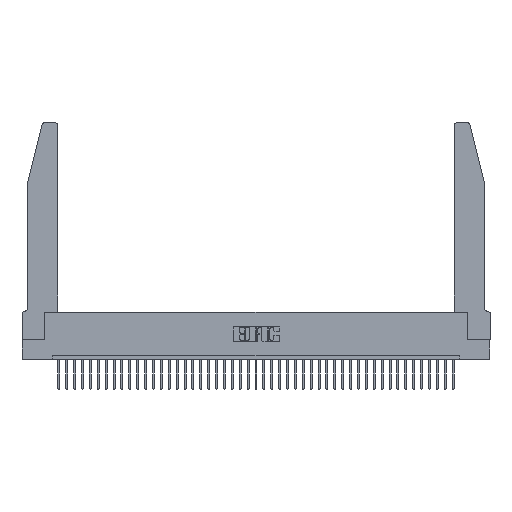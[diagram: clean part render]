
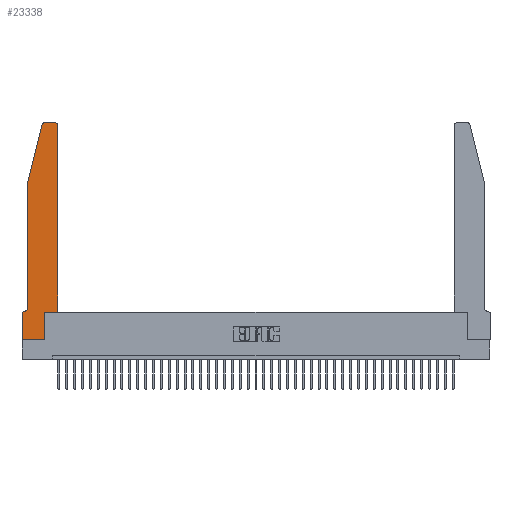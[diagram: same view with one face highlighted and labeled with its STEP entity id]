
A CAD part, top view. The second image highlights one B-rep face of the part: STEP entity #23338.
In plain terms, the highlighted planar face has unit normal (0, 0, 1).
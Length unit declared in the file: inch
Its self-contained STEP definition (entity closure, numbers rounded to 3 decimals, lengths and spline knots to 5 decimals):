
#655 = VERTEX_POINT ( 'NONE', #18500 ) ;
#844 = EDGE_CURVE ( 'NONE', #29490, #19747, #3680, .T. ) ;
#897 = DIRECTION ( 'NONE',  ( 0., -1., 0. ) ) ;
#1225 = VERTEX_POINT ( 'NONE', #5755 ) ;
#1467 = FACE_OUTER_BOUND ( 'NONE', #24844, .T. ) ;
#1492 = DIRECTION ( 'NONE',  ( 0., 0., 1. ) ) ;
#1796 = CARTESIAN_POINT ( 'NONE',  ( 0.284, 2.75, 0.37 ) ) ;
#1961 = CARTESIAN_POINT ( 'NONE',  ( 0.0755, 2., 0.37 ) ) ;
#2052 = VERTEX_POINT ( 'NONE', #10252 ) ;
#2252 = VECTOR ( 'NONE', #21838, 39.37008 ) ;
#2318 = CARTESIAN_POINT ( 'NONE',  ( 0.2605, 2.75, 0.37 ) ) ;
#2495 = VECTOR ( 'NONE', #20923, 39.37008 ) ;
#2794 = ORIENTED_EDGE ( 'NONE', *, *, #21121, .T. ) ;
#3680 = CIRCLE ( 'NONE', #6581, 0.03 ) ;
#4065 = CARTESIAN_POINT ( 'NONE',  ( 0., 0., 0.37 ) ) ;
#4233 = VECTOR ( 'NONE', #21711, 39.37008 ) ;
#5175 = CARTESIAN_POINT ( 'NONE',  ( 0.4505, 0.35, 0.37 ) ) ;
#5755 = CARTESIAN_POINT ( 'NONE',  ( 0.2865, 0.35, 0.37 ) ) ;
#6344 = LINE ( 'NONE', #2318, #2252 ) ;
#6581 = AXIS2_PLACEMENT_3D ( 'NONE', #23271, #13823, #37206 ) ;
#7173 = VERTEX_POINT ( 'NONE', #1796 ) ;
#7317 = LINE ( 'NONE', #12510, #4233 ) ;
#7359 = ORIENTED_EDGE ( 'NONE', *, *, #10147, .T. ) ;
#7855 = ORIENTED_EDGE ( 'NONE', *, *, #9364, .T. ) ;
#8074 = DIRECTION ( 'NONE',  ( 1., 0., 0. ) ) ;
#8273 = ORIENTED_EDGE ( 'NONE', *, *, #15355, .T. ) ;
#8410 = CARTESIAN_POINT ( 'NONE',  ( 0.4505, 0.35, 0.37 ) ) ;
#9364 = EDGE_CURVE ( 'NONE', #10448, #33351, #32750, .T. ) ;
#9763 = CARTESIAN_POINT ( 'NONE',  ( 0.284, 2.72, 0.37 ) ) ;
#10147 = EDGE_CURVE ( 'NONE', #38852, #29490, #27748, .T. ) ;
#10252 = CARTESIAN_POINT ( 'NONE',  ( 0.25487, 2.72718, 0.37 ) ) ;
#10448 = VERTEX_POINT ( 'NONE', #26435 ) ;
#11388 = VERTEX_POINT ( 'NONE', #17758 ) ;
#12142 = ORIENTED_EDGE ( 'NONE', *, *, #20381, .T. ) ;
#12510 = CARTESIAN_POINT ( 'NONE',  ( 0.0755, 2., 0.37 ) ) ;
#12698 = DIRECTION ( 'NONE',  ( 0., 1., 0. ) ) ;
#13823 = DIRECTION ( 'NONE',  ( 0., 0., 1. ) ) ;
#13905 = DIRECTION ( 'NONE',  ( 0., 0., 1. ) ) ;
#13908 = PLANE ( 'NONE',  #20901 ) ;
#14252 = LINE ( 'NONE', #28905, #28902 ) ;
#14485 = ORIENTED_EDGE ( 'NONE', *, *, #21116, .T. ) ;
#14889 = CARTESIAN_POINT ( 'NONE',  ( 0.4205, 2.75, 0.37 ) ) ;
#14927 = EDGE_CURVE ( 'NONE', #7173, #2052, #18191, .T. ) ;
#15355 = EDGE_CURVE ( 'NONE', #2052, #39242, #28479, .T. ) ;
#15704 = AXIS2_PLACEMENT_3D ( 'NONE', #33515, #37366, #37084 ) ;
#16388 = LINE ( 'NONE', #5175, #30599 ) ;
#17758 = CARTESIAN_POINT ( 'NONE',  ( 0.0755, 0.42, 0.37 ) ) ;
#18191 = CIRCLE ( 'NONE', #26035, 0.03 ) ;
#18500 = CARTESIAN_POINT ( 'NONE',  ( 0.0055, 0.35, 0.37 ) ) ;
#19199 = ORIENTED_EDGE ( 'NONE', *, *, #26691, .T. ) ;
#19747 = VERTEX_POINT ( 'NONE', #14889 ) ;
#20086 = DIRECTION ( 'NONE',  ( 1., 0., 0. ) ) ;
#20381 = EDGE_CURVE ( 'NONE', #11388, #655, #41296, .T. ) ;
#20901 = AXIS2_PLACEMENT_3D ( 'NONE', #23945, #1492, #8074 ) ;
#20923 = DIRECTION ( 'NONE',  ( 0., 1., 0. ) ) ;
#21116 = EDGE_CURVE ( 'NONE', #39242, #11388, #7317, .T. ) ;
#21121 = EDGE_CURVE ( 'NONE', #19747, #7173, #6344, .T. ) ;
#21711 = DIRECTION ( 'NONE',  ( 0., -1., 0. ) ) ;
#21838 = DIRECTION ( 'NONE',  ( -1., 0., 0. ) ) ;
#23271 = CARTESIAN_POINT ( 'NONE',  ( 0.4205, 2.72, 0.37 ) ) ;
#23338 = ADVANCED_FACE ( 'NONE', ( #1467 ), #13908, .T. ) ;
#23424 = CARTESIAN_POINT ( 'NONE',  ( 0., 0., 0.37 ) ) ;
#23945 = CARTESIAN_POINT ( 'NONE',  ( 0., 0.35, 0.37 ) ) ;
#24200 = VECTOR ( 'NONE', #897, 39.37008 ) ;
#24362 = DIRECTION ( 'NONE',  ( 1., 0., 0. ) ) ;
#24666 = ORIENTED_EDGE ( 'NONE', *, *, #38622, .T. ) ;
#24844 = EDGE_LOOP ( 'NONE', ( #2794, #31527, #8273, #14485, #12142, #19199, #7855, #34890, #40819, #24666, #7359, #34137 ) ) ;
#25403 = CARTESIAN_POINT ( 'NONE',  ( 0.0755, 0.35, 0.37 ) ) ;
#26035 = AXIS2_PLACEMENT_3D ( 'NONE', #9763, #13905, #20086 ) ;
#26435 = CARTESIAN_POINT ( 'NONE',  ( 0., 0.35, 0.37 ) ) ;
#26639 = EDGE_CURVE ( 'NONE', #29148, #1225, #14252, .T. ) ;
#26691 = EDGE_CURVE ( 'NONE', #655, #10448, #41616, .T. ) ;
#27676 = EDGE_CURVE ( 'NONE', #33351, #29148, #29787, .T. ) ;
#27748 = LINE ( 'NONE', #8410, #2495 ) ;
#28479 = LINE ( 'NONE', #1961, #36472 ) ;
#28902 = VECTOR ( 'NONE', #12698, 39.37008 ) ;
#28905 = CARTESIAN_POINT ( 'NONE',  ( 0.2865, 0.35, 0.37 ) ) ;
#29148 = VERTEX_POINT ( 'NONE', #35336 ) ;
#29490 = VERTEX_POINT ( 'NONE', #30052 ) ;
#29787 = LINE ( 'NONE', #38335, #36433 ) ;
#30015 = DIRECTION ( 'NONE',  ( -1., 0., 0. ) ) ;
#30052 = CARTESIAN_POINT ( 'NONE',  ( 0.4505, 2.72, 0.37 ) ) ;
#30215 = CARTESIAN_POINT ( 'NONE',  ( 0.4505, 0.35, 0.37 ) ) ;
#30599 = VECTOR ( 'NONE', #24362, 39.37008 ) ;
#31393 = DIRECTION ( 'NONE',  ( 1., 0., 0. ) ) ;
#31527 = ORIENTED_EDGE ( 'NONE', *, *, #14927, .T. ) ;
#31965 = VECTOR ( 'NONE', #30015, 39.37008 ) ;
#32750 = LINE ( 'NONE', #23424, #24200 ) ;
#33351 = VERTEX_POINT ( 'NONE', #4065 ) ;
#33515 = CARTESIAN_POINT ( 'NONE',  ( 0.0055, 0.42, 0.37 ) ) ;
#34137 = ORIENTED_EDGE ( 'NONE', *, *, #844, .T. ) ;
#34890 = ORIENTED_EDGE ( 'NONE', *, *, #27676, .T. ) ;
#35336 = CARTESIAN_POINT ( 'NONE',  ( 0.2865, 0., 0.37 ) ) ;
#36433 = VECTOR ( 'NONE', #31393, 39.37008 ) ;
#36472 = VECTOR ( 'NONE', #40980, 39.37008 ) ;
#37084 = DIRECTION ( 'NONE',  ( -1., 0., 0. ) ) ;
#37206 = DIRECTION ( 'NONE',  ( 1., 0., 0. ) ) ;
#37366 = DIRECTION ( 'NONE',  ( 0., 0., -1. ) ) ;
#38335 = CARTESIAN_POINT ( 'NONE',  ( 0., 0., 0.37 ) ) ;
#38622 = EDGE_CURVE ( 'NONE', #1225, #38852, #16388, .T. ) ;
#38852 = VERTEX_POINT ( 'NONE', #30215 ) ;
#39064 = CARTESIAN_POINT ( 'NONE',  ( 0.0755, 2., 0.37 ) ) ;
#39242 = VERTEX_POINT ( 'NONE', #39064 ) ;
#40819 = ORIENTED_EDGE ( 'NONE', *, *, #26639, .T. ) ;
#40980 = DIRECTION ( 'NONE',  ( -0.239, -0.971, 0. ) ) ;
#41296 = CIRCLE ( 'NONE', #15704, 0.07 ) ;
#41616 = LINE ( 'NONE', #25403, #31965 ) ;
